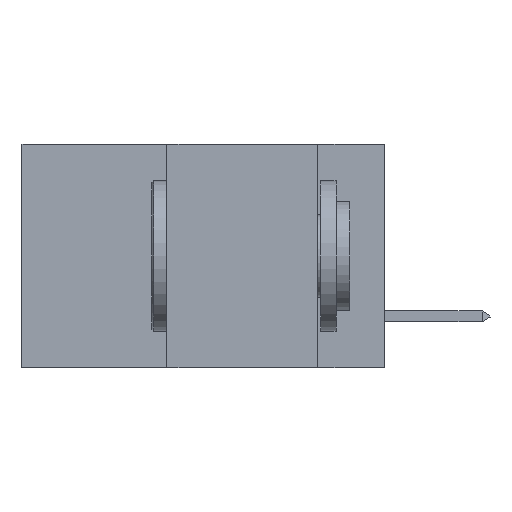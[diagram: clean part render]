
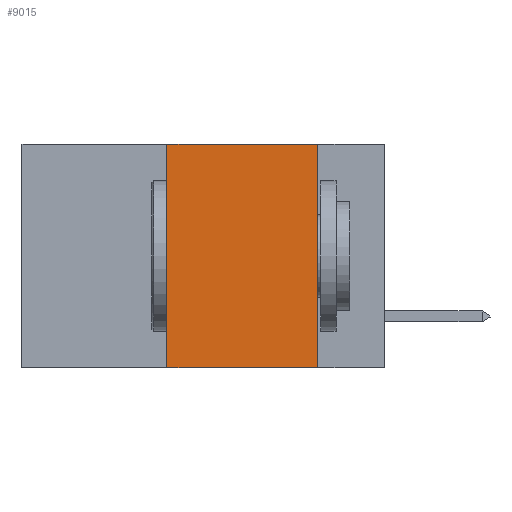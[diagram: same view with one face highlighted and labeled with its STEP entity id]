
A CAD part, left-side view. The second image highlights one B-rep face of the part: STEP entity #9015.
In plain terms, the highlighted planar face has unit normal (-1, 0, 0).
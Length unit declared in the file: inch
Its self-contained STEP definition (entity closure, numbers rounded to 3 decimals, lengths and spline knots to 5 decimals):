
#410 = CARTESIAN_POINT ( 'NONE',  ( 0., 0.36, 0. ) ) ;
#430 = ORIENTED_EDGE ( 'NONE', *, *, #8661, .F. ) ;
#811 = CARTESIAN_POINT ( 'NONE',  ( 0., 0.6, 0. ) ) ;
#1228 = ORIENTED_EDGE ( 'NONE', *, *, #12700, .F. ) ;
#1704 = DIRECTION ( 'NONE',  ( 0., 0., 1. ) ) ;
#2473 = CARTESIAN_POINT ( 'NONE',  ( 0., 0.36, 0. ) ) ;
#2598 = LINE ( 'NONE', #410, #12482 ) ;
#2848 = PLANE ( 'NONE',  #9964 ) ;
#3511 = CARTESIAN_POINT ( 'NONE',  ( 0., 0.11, 0. ) ) ;
#4203 = DIRECTION ( 'NONE',  ( 0., 0., -1. ) ) ;
#4947 = LINE ( 'NONE', #8667, #14644 ) ;
#5951 = DIRECTION ( 'NONE',  ( 0., -1., 0. ) ) ;
#7190 = CARTESIAN_POINT ( 'NONE',  ( 0., 0.36, -0.37 ) ) ;
#7918 = VECTOR ( 'NONE', #9896, 39.37008 ) ;
#8064 = CARTESIAN_POINT ( 'NONE',  ( 0., 0.6, 0. ) ) ;
#8182 = VERTEX_POINT ( 'NONE', #12723 ) ;
#8188 = VERTEX_POINT ( 'NONE', #2473 ) ;
#8291 = VECTOR ( 'NONE', #5951, 39.37008 ) ;
#8661 = EDGE_CURVE ( 'NONE', #10566, #8182, #4947, .T. ) ;
#8667 = CARTESIAN_POINT ( 'NONE',  ( 0., 0.11, 0. ) ) ;
#9015 = ADVANCED_FACE ( 'NONE', ( #15946 ), #2848, .F. ) ;
#9783 = VERTEX_POINT ( 'NONE', #7190 ) ;
#9893 = DIRECTION ( 'NONE',  ( 0., 0., -1. ) ) ;
#9896 = DIRECTION ( 'NONE',  ( 0., -1., 0. ) ) ;
#9964 = AXIS2_PLACEMENT_3D ( 'NONE', #8064, #11864, #4203 ) ;
#10566 = VERTEX_POINT ( 'NONE', #3511 ) ;
#11187 = LINE ( 'NONE', #13519, #8291 ) ;
#11864 = DIRECTION ( 'NONE',  ( 1., 0., 0. ) ) ;
#11948 = ORIENTED_EDGE ( 'NONE', *, *, #16369, .F. ) ;
#12482 = VECTOR ( 'NONE', #1704, 39.37008 ) ;
#12700 = EDGE_CURVE ( 'NONE', #8188, #10566, #14893, .T. ) ;
#12723 = CARTESIAN_POINT ( 'NONE',  ( 0., 0.11, -0.37 ) ) ;
#13177 = EDGE_CURVE ( 'NONE', #9783, #8182, #11187, .T. ) ;
#13519 = CARTESIAN_POINT ( 'NONE',  ( 0., 0.6, -0.37 ) ) ;
#14644 = VECTOR ( 'NONE', #9893, 39.37008 ) ;
#14893 = LINE ( 'NONE', #811, #7918 ) ;
#15580 = ORIENTED_EDGE ( 'NONE', *, *, #13177, .T. ) ;
#15946 = FACE_OUTER_BOUND ( 'NONE', #16418, .T. ) ;
#16369 = EDGE_CURVE ( 'NONE', #9783, #8188, #2598, .T. ) ;
#16418 = EDGE_LOOP ( 'NONE', ( #430, #1228, #11948, #15580 ) ) ;
